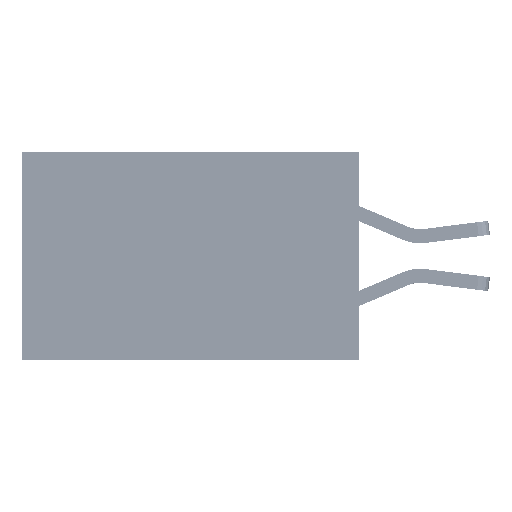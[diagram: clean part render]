
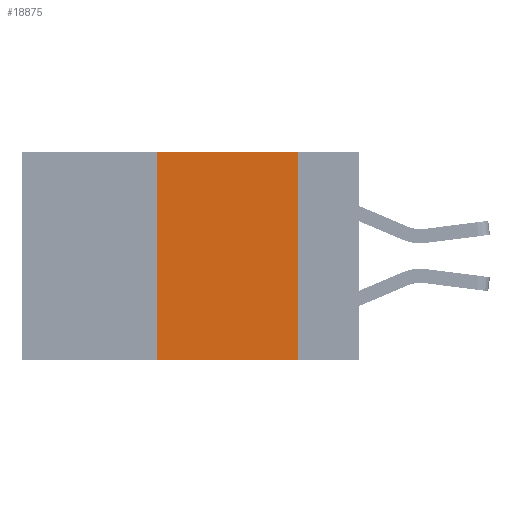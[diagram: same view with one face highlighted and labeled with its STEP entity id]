
A CAD part, left-side view. The second image highlights one B-rep face of the part: STEP entity #18875.
In plain terms, the highlighted planar face has unit normal (-1, 0, 0).
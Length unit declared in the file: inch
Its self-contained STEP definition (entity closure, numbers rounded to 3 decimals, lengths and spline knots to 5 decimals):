
#2990 = DIRECTION ( 'NONE',  ( 0., 0., 1. ) ) ;
#5047 = LINE ( 'NONE', #43050, #38666 ) ;
#5244 = EDGE_CURVE ( 'NONE', #18090, #13572, #17925, .T. ) ;
#6543 = ORIENTED_EDGE ( 'NONE', *, *, #5244, .F. ) ;
#9631 = DIRECTION ( 'NONE',  ( 0., 0., -1. ) ) ;
#10627 = CARTESIAN_POINT ( 'NONE',  ( 0., 0.36, -0.37 ) ) ;
#11587 = VERTEX_POINT ( 'NONE', #49968 ) ;
#12259 = EDGE_CURVE ( 'NONE', #11587, #18090, #30378, .T. ) ;
#13572 = VERTEX_POINT ( 'NONE', #39197 ) ;
#14287 = PLANE ( 'NONE',  #51593 ) ;
#14638 = DIRECTION ( 'NONE',  ( 0., 0., -1. ) ) ;
#15984 = VECTOR ( 'NONE', #48091, 39.37008 ) ;
#17925 = LINE ( 'NONE', #45913, #36023 ) ;
#18090 = VERTEX_POINT ( 'NONE', #25345 ) ;
#18110 = DIRECTION ( 'NONE',  ( 1., 0., 0. ) ) ;
#18820 = VERTEX_POINT ( 'NONE', #10627 ) ;
#18875 = ADVANCED_FACE ( 'NONE', ( #42599 ), #14287, .F. ) ;
#22734 = EDGE_CURVE ( 'NONE', #18820, #11587, #37634, .T. ) ;
#25345 = CARTESIAN_POINT ( 'NONE',  ( 0., 0.11, 0. ) ) ;
#26410 = VECTOR ( 'NONE', #2990, 39.37008 ) ;
#29529 = ORIENTED_EDGE ( 'NONE', *, *, #22734, .F. ) ;
#30378 = LINE ( 'NONE', #50736, #15984 ) ;
#32212 = ORIENTED_EDGE ( 'NONE', *, *, #12259, .F. ) ;
#34468 = CARTESIAN_POINT ( 'NONE',  ( 0., 0.6, 0. ) ) ;
#34996 = CARTESIAN_POINT ( 'NONE',  ( 0., 0.36, 0. ) ) ;
#36023 = VECTOR ( 'NONE', #9631, 39.37008 ) ;
#37634 = LINE ( 'NONE', #34996, #26410 ) ;
#37777 = EDGE_CURVE ( 'NONE', #18820, #13572, #5047, .T. ) ;
#38666 = VECTOR ( 'NONE', #47234, 39.37008 ) ;
#39197 = CARTESIAN_POINT ( 'NONE',  ( 0., 0.11, -0.37 ) ) ;
#42072 = ORIENTED_EDGE ( 'NONE', *, *, #37777, .T. ) ;
#42599 = FACE_OUTER_BOUND ( 'NONE', #44601, .T. ) ;
#43050 = CARTESIAN_POINT ( 'NONE',  ( 0., 0.6, -0.37 ) ) ;
#44601 = EDGE_LOOP ( 'NONE', ( #6543, #32212, #29529, #42072 ) ) ;
#45913 = CARTESIAN_POINT ( 'NONE',  ( 0., 0.11, 0. ) ) ;
#47234 = DIRECTION ( 'NONE',  ( 0., -1., 0. ) ) ;
#48091 = DIRECTION ( 'NONE',  ( 0., -1., 0. ) ) ;
#49968 = CARTESIAN_POINT ( 'NONE',  ( 0., 0.36, 0. ) ) ;
#50736 = CARTESIAN_POINT ( 'NONE',  ( 0., 0.6, 0. ) ) ;
#51593 = AXIS2_PLACEMENT_3D ( 'NONE', #34468, #18110, #14638 ) ;
